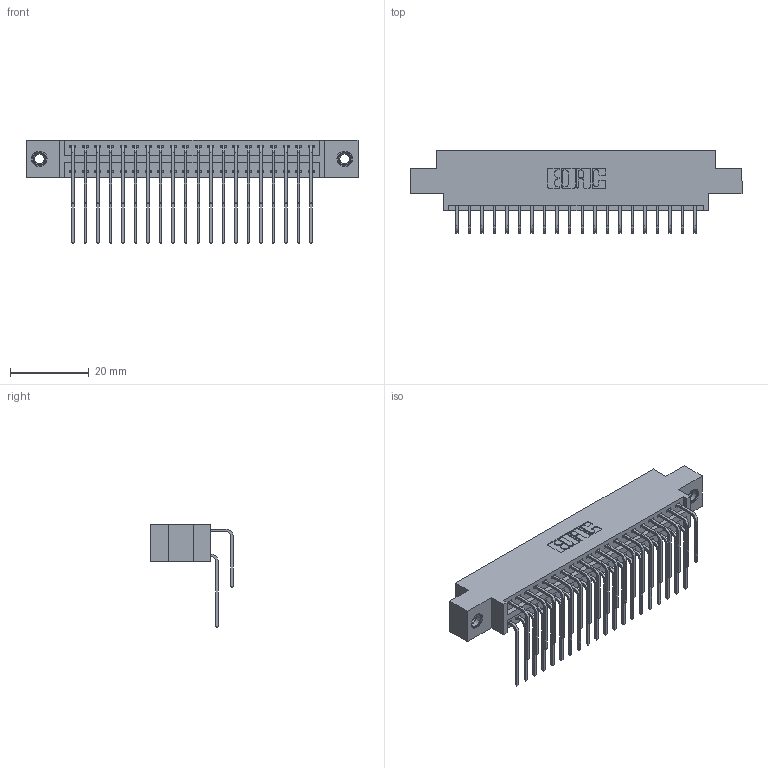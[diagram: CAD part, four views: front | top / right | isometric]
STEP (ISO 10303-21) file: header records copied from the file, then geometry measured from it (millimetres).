
FILE_DESCRIPTION (( 'STEP AP203' ), '1' );
FILE_NAME ('396-040-559-807.STEP', '2019-11-03T07:35:13', ( '' ), ( '' ), 'SwSTEP 2.0', 'SolidWorks 2016', '' );
FILE_SCHEMA (( 'CONFIG_CONTROL_DESIGN' ));
Length unit declared in the file: inch
Products named in the file (5): 345-292-001_559 Tail - 2; 345-250-001_345-250-005-103; 346 Part_0.170 Offset - 0.156 Dia-TI; 345-292-001_558 559 Tail - 1; 396-040-559-807
Assembly tree (43 placements, depth 2):
  396-040-559-807
    346 Part_0.170 Offset - 0.156 Dia-TI
    345-292-001_558 559 Tail - 1  x20
    345-292-001_559 Tail - 2  x20
    345-250-001_345-250-005-103  x2
Bounding box: 84.07 x 20.89 x 26.16 mm (x, y, z)
Volume: 8090 mm3; surface area: 12094.8 mm2
Topology: 43 solids, 43 shells, 2346 faces, 6917 edges, 4550 vertices
Faces by surface type: plane 1592, cylinder 738, cone 12, torus 4
Entity records: 19116 total; most frequent: CARTESIAN_POINT 3218, ORIENTED_EDGE 3094, DIRECTION 2885, EDGE_CURVE 1547, VECTOR 1275, LINE 1275, VERTEX_POINT 1024, AXIS2_PLACEMENT_3D 805
